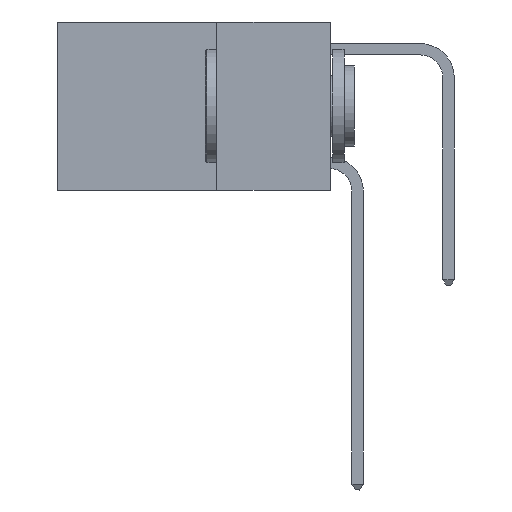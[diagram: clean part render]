
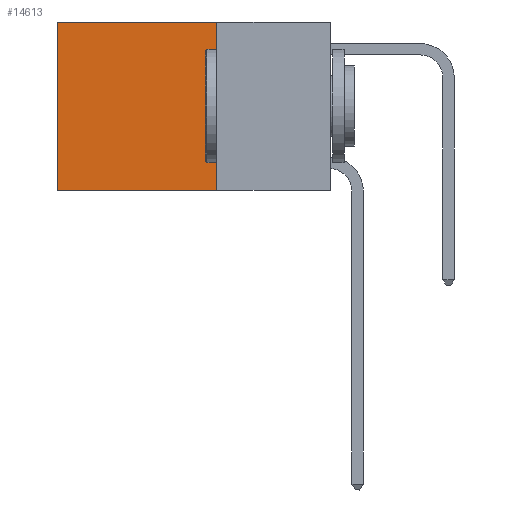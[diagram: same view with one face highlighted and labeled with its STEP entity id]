
A CAD part, left-side view. The second image highlights one B-rep face of the part: STEP entity #14613.
In plain terms, the highlighted planar face has unit normal (-1, 0, 0).
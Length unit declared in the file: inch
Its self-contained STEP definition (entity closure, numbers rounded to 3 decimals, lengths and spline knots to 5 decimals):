
#302 = DIRECTION ( 'NONE',  ( 0., 0., -1. ) ) ;
#849 = VECTOR ( 'NONE', #6583, 39.37008 ) ;
#3046 = VECTOR ( 'NONE', #25132, 39.37008 ) ;
#4623 = DIRECTION ( 'NONE',  ( 0., 1., 0. ) ) ;
#4636 = CARTESIAN_POINT ( 'NONE',  ( 0.2625, 0.6, 0. ) ) ;
#4803 = CARTESIAN_POINT ( 'NONE',  ( 0.2625, 0.25, 0. ) ) ;
#5065 = ORIENTED_EDGE ( 'NONE', *, *, #8340, .F. ) ;
#6583 = DIRECTION ( 'NONE',  ( 0., 0., -1. ) ) ;
#7384 = EDGE_CURVE ( 'NONE', #12221, #19343, #24626, .T. ) ;
#7867 = ORIENTED_EDGE ( 'NONE', *, *, #19296, .T. ) ;
#8340 = EDGE_CURVE ( 'NONE', #9124, #12221, #29086, .T. ) ;
#9124 = VERTEX_POINT ( 'NONE', #21647 ) ;
#12221 = VERTEX_POINT ( 'NONE', #20911 ) ;
#12774 = ORIENTED_EDGE ( 'NONE', *, *, #22742, .T. ) ;
#13401 = CARTESIAN_POINT ( 'NONE',  ( 0.2625, 0.6, -0.37 ) ) ;
#13911 = VECTOR ( 'NONE', #24928, 39.37008 ) ;
#14613 = ADVANCED_FACE ( 'NONE', ( #18405 ), #27575, .F. ) ;
#16011 = AXIS2_PLACEMENT_3D ( 'NONE', #25642, #22996, #302 ) ;
#16594 = CARTESIAN_POINT ( 'NONE',  ( 0.2625, 0.6, 0. ) ) ;
#17976 = EDGE_LOOP ( 'NONE', ( #7867, #24432, #5065, #12774 ) ) ;
#18320 = LINE ( 'NONE', #25805, #3046 ) ;
#18405 = FACE_OUTER_BOUND ( 'NONE', #17976, .T. ) ;
#18822 = VERTEX_POINT ( 'NONE', #16594 ) ;
#19296 = EDGE_CURVE ( 'NONE', #18822, #19343, #27153, .T. ) ;
#19343 = VERTEX_POINT ( 'NONE', #13401 ) ;
#20911 = CARTESIAN_POINT ( 'NONE',  ( 0.2625, 0.25, -0.37 ) ) ;
#21647 = CARTESIAN_POINT ( 'NONE',  ( 0.2625, 0.25, 0. ) ) ;
#22742 = EDGE_CURVE ( 'NONE', #9124, #18822, #18320, .T. ) ;
#22996 = DIRECTION ( 'NONE',  ( 1., 0., 0. ) ) ;
#24432 = ORIENTED_EDGE ( 'NONE', *, *, #7384, .F. ) ;
#24626 = LINE ( 'NONE', #24915, #25498 ) ;
#24915 = CARTESIAN_POINT ( 'NONE',  ( 0.2625, 0.25, -0.37 ) ) ;
#24928 = DIRECTION ( 'NONE',  ( 0., 0., -1. ) ) ;
#25132 = DIRECTION ( 'NONE',  ( 0., 1., 0. ) ) ;
#25498 = VECTOR ( 'NONE', #4623, 39.37008 ) ;
#25642 = CARTESIAN_POINT ( 'NONE',  ( 0.2625, 0.25, 0. ) ) ;
#25805 = CARTESIAN_POINT ( 'NONE',  ( 0.2625, 0.25, 0. ) ) ;
#27153 = LINE ( 'NONE', #4636, #13911 ) ;
#27575 = PLANE ( 'NONE',  #16011 ) ;
#29086 = LINE ( 'NONE', #4803, #849 ) ;
